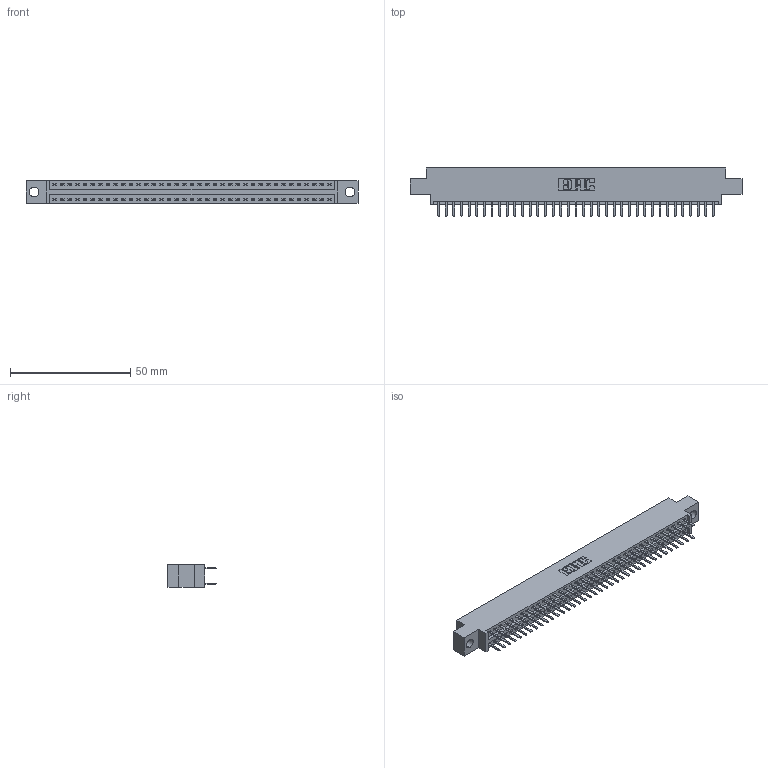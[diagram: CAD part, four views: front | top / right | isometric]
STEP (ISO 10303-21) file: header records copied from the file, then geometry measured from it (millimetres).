
FILE_DESCRIPTION (( 'STEP AP203' ), '1' );
FILE_NAME ('346-074-520-804.STEP', '2022-05-25T01:43:33', ( '' ), ( '' ), 'SwSTEP 2.0', 'SolidWorks 2020', '' );
FILE_SCHEMA (( 'CONFIG_CONTROL_DESIGN' ));
Length unit declared in the file: inch
Products named in the file (3): 346-074-520-804; 346 Part_0.170 Offset - 0.156 Dia-TH; 345-292-001_345-293-120
Assembly tree (75 placements, depth 2):
  346-074-520-804
    346 Part_0.170 Offset - 0.156 Dia-TH
    345-292-001_345-293-120  x74
Bounding box: 138.05 x 20.02 x 9.4 mm (x, y, z)
Volume: 13129.6 mm3; surface area: 17920.2 mm2
Topology: 75 solids, 75 shells, 4284 faces, 12439 edges, 8094 vertices
Faces by surface type: plane 2832, cylinder 1452
Entity records: 25485 total; most frequent: CARTESIAN_POINT 4226, ORIENTED_EDGE 4146, DIRECTION 3761, EDGE_CURVE 2073, VECTOR 1789, LINE 1789, VERTEX_POINT 1378, AXIS2_PLACEMENT_3D 986
